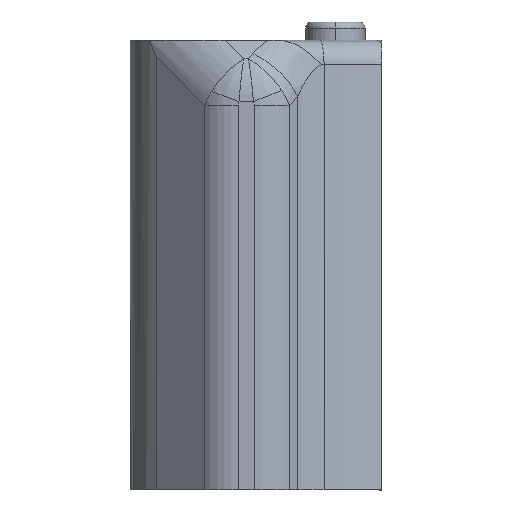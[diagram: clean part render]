
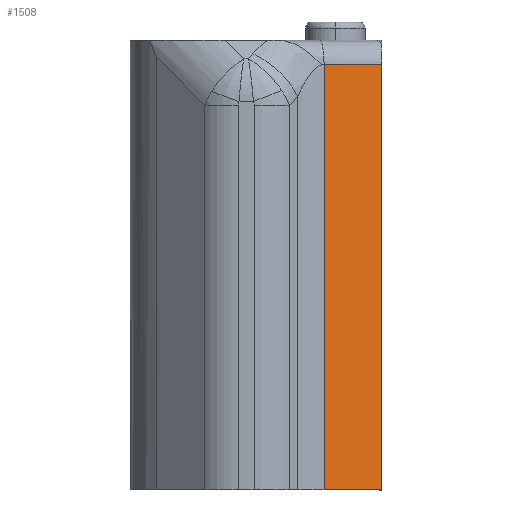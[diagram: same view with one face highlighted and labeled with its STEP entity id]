
A CAD part, left-side view. The second image highlights one B-rep face of the part: STEP entity #1508.
In plain terms, the highlighted cylindrical face has radius 35 mm (diameter 70 mm), a partial arc.
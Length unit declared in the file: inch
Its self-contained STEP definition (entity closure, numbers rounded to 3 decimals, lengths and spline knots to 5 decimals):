
#1 = CIRCLE ( 'NONE', #1740, 1.37795 ) ;
#5 = EDGE_CURVE ( 'NONE', #895, #1672, #1, .T. ) ;
#89 = DIRECTION ( 'NONE',  ( -1., 0., 0. ) ) ;
#90 = CARTESIAN_POINT ( 'NONE',  ( 5.62236, 6.96053, 5.09136 ) ) ;
#99 = CYLINDRICAL_SURFACE ( 'NONE', #1772, 1.37795 ) ;
#119 = CIRCLE ( 'NONE', #1783, 1.37795 ) ;
#188 = LINE ( 'NONE', #493, #875 ) ;
#212 = EDGE_CURVE ( 'NONE', #1672, #1802, #333, .T. ) ;
#297 = FACE_OUTER_BOUND ( 'NONE', #1897, .T. ) ;
#330 = VECTOR ( 'NONE', #2156, 39.37008 ) ;
#333 = LINE ( 'NONE', #2191, #330 ) ;
#459 = DIRECTION ( 'NONE',  ( 0., 0., 1. ) ) ;
#493 = CARTESIAN_POINT ( 'NONE',  ( 4.4583, 6.22317, 12.08462 ) ) ;
#514 = CARTESIAN_POINT ( 'NONE',  ( 4.4583, 6.22317, 5.09136 ) ) ;
#621 = CARTESIAN_POINT ( 'NONE',  ( 4.26914, 6.70065, 8.61076 ) ) ;
#637 = CARTESIAN_POINT ( 'NONE',  ( 4.26914, 6.70065, 5.09136 ) ) ;
#764 = EDGE_CURVE ( 'NONE', #1802, #1961, #119, .T. ) ;
#772 = ORIENTED_EDGE ( 'NONE', *, *, #212, .T. ) ;
#875 = VECTOR ( 'NONE', #459, 39.37008 ) ;
#895 = VERTEX_POINT ( 'NONE', #2094 ) ;
#941 = DIRECTION ( 'NONE',  ( 1., 0., 0. ) ) ;
#970 = DIRECTION ( 'NONE',  ( 0., 0., 1. ) ) ;
#972 = CARTESIAN_POINT ( 'NONE',  ( 5.62236, 6.96053, 12.08462 ) ) ;
#1035 = ORIENTED_EDGE ( 'NONE', *, *, #5, .T. ) ;
#1048 = ORIENTED_EDGE ( 'NONE', *, *, #764, .T. ) ;
#1443 = ORIENTED_EDGE ( 'NONE', *, *, #2082, .T. ) ;
#1508 = ADVANCED_FACE ( 'NONE', ( #297 ), #99, .T. ) ;
#1672 = VERTEX_POINT ( 'NONE', #621 ) ;
#1740 = AXIS2_PLACEMENT_3D ( 'NONE', #2052, #1999, #1820 ) ;
#1772 = AXIS2_PLACEMENT_3D ( 'NONE', #972, #970, #941 ) ;
#1783 = AXIS2_PLACEMENT_3D ( 'NONE', #90, #2184, #89 ) ;
#1802 = VERTEX_POINT ( 'NONE', #637 ) ;
#1820 = DIRECTION ( 'NONE',  ( 1., 0., 0. ) ) ;
#1897 = EDGE_LOOP ( 'NONE', ( #772, #1048, #1443, #1035 ) ) ;
#1961 = VERTEX_POINT ( 'NONE', #514 ) ;
#1999 = DIRECTION ( 'NONE',  ( 0., 0., -1. ) ) ;
#2052 = CARTESIAN_POINT ( 'NONE',  ( 5.62236, 6.96053, 8.61076 ) ) ;
#2082 = EDGE_CURVE ( 'NONE', #1961, #895, #188, .T. ) ;
#2094 = CARTESIAN_POINT ( 'NONE',  ( 4.4583, 6.22317, 8.61076 ) ) ;
#2156 = DIRECTION ( 'NONE',  ( 0., 0., -1. ) ) ;
#2184 = DIRECTION ( 'NONE',  ( 0., 0., 1. ) ) ;
#2191 = CARTESIAN_POINT ( 'NONE',  ( 4.26914, 6.70065, 12.08462 ) ) ;
